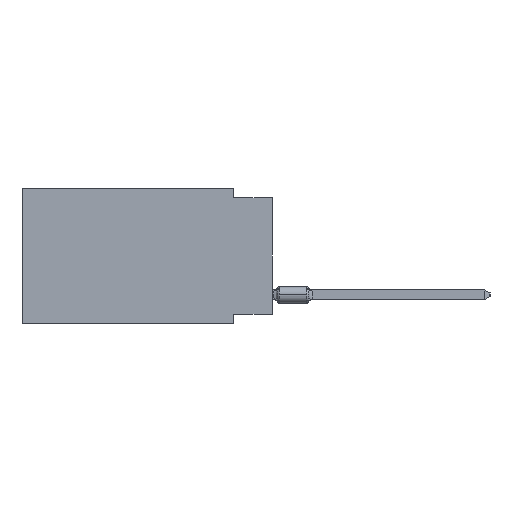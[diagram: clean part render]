
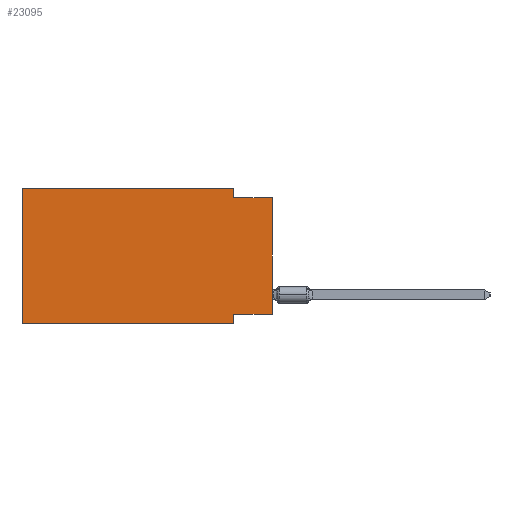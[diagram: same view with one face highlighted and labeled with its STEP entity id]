
A CAD part, left-side view. The second image highlights one B-rep face of the part: STEP entity #23095.
In plain terms, the highlighted planar face has unit normal (-1, 0, 0).
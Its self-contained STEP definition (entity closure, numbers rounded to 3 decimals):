
#144 = EDGE_CURVE ( 'NONE', #15184, #32745, #8594, .T. ) ;
#455 = ORIENTED_EDGE ( 'NONE', *, *, #16680, .F. ) ;
#2168 = ORIENTED_EDGE ( 'NONE', *, *, #20220, .F. ) ;
#2653 = CARTESIAN_POINT ( 'NONE',  ( 0., 0., -0.635 ) ) ;
#5180 = LINE ( 'NONE', #40869, #28693 ) ;
#6357 = ORIENTED_EDGE ( 'NONE', *, *, #12459, .T. ) ;
#7668 = DIRECTION ( 'NONE',  ( 0., 0., -1. ) ) ;
#8041 = ORIENTED_EDGE ( 'NONE', *, *, #144, .F. ) ;
#8301 = CARTESIAN_POINT ( 'NONE',  ( 0., 16.383, 0. ) ) ;
#8594 = LINE ( 'NONE', #16856, #38137 ) ;
#9159 = LINE ( 'NONE', #21857, #26426 ) ;
#9994 = VERTEX_POINT ( 'NONE', #51847 ) ;
#10965 = VECTOR ( 'NONE', #41348, 1000. ) ;
#11211 = CARTESIAN_POINT ( 'NONE',  ( 0., 2.54, 0. ) ) ;
#11856 = VERTEX_POINT ( 'NONE', #39133 ) ;
#12459 = EDGE_CURVE ( 'NONE', #15184, #53802, #41325, .T. ) ;
#12996 = DIRECTION ( 'NONE',  ( 0., 0., -1. ) ) ;
#15184 = VERTEX_POINT ( 'NONE', #36613 ) ;
#15350 = EDGE_LOOP ( 'NONE', ( #41732, #2168, #28341, #30673, #8041, #6357, #15397, #455 ) ) ;
#15397 = ORIENTED_EDGE ( 'NONE', *, *, #29997, .F. ) ;
#15806 = CARTESIAN_POINT ( 'NONE',  ( 0., 0., -8.255 ) ) ;
#16680 = EDGE_CURVE ( 'NONE', #45588, #11856, #53089, .T. ) ;
#16856 = CARTESIAN_POINT ( 'NONE',  ( 0., 16.383, 0. ) ) ;
#17795 = VECTOR ( 'NONE', #7668, 1000. ) ;
#18474 = AXIS2_PLACEMENT_3D ( 'NONE', #33697, #32548, #50539 ) ;
#18913 = DIRECTION ( 'NONE',  ( 0., -1., 0. ) ) ;
#20220 = EDGE_CURVE ( 'NONE', #9994, #50103, #5180, .T. ) ;
#21504 = VECTOR ( 'NONE', #18913, 1000. ) ;
#21857 = CARTESIAN_POINT ( 'NONE',  ( 0., 2.54, -8.89 ) ) ;
#21991 = CARTESIAN_POINT ( 'NONE',  ( 0., 2.54, 0. ) ) ;
#22128 = DIRECTION ( 'NONE',  ( 0., 1., 0. ) ) ;
#23095 = ADVANCED_FACE ( 'NONE', ( #55823 ), #23418, .F. ) ;
#23418 = PLANE ( 'NONE',  #18474 ) ;
#23949 = LINE ( 'NONE', #45471, #10965 ) ;
#26426 = VECTOR ( 'NONE', #12996, 1000. ) ;
#26551 = CARTESIAN_POINT ( 'NONE',  ( 0., 0., -8.255 ) ) ;
#27230 = EDGE_CURVE ( 'NONE', #45695, #9994, #56624, .T. ) ;
#27297 = CARTESIAN_POINT ( 'NONE',  ( 0., 0., 0. ) ) ;
#28169 = DIRECTION ( 'NONE',  ( 0., -1., 0. ) ) ;
#28341 = ORIENTED_EDGE ( 'NONE', *, *, #27230, .F. ) ;
#28693 = VECTOR ( 'NONE', #28169, 1000. ) ;
#29997 = EDGE_CURVE ( 'NONE', #11856, #53802, #9159, .T. ) ;
#30673 = ORIENTED_EDGE ( 'NONE', *, *, #43384, .F. ) ;
#30845 = DIRECTION ( 'NONE',  ( 0., 0., 1. ) ) ;
#31423 = LINE ( 'NONE', #27297, #57673 ) ;
#32055 = VECTOR ( 'NONE', #22128, 1000. ) ;
#32548 = DIRECTION ( 'NONE',  ( 1., 0., 0. ) ) ;
#32745 = VERTEX_POINT ( 'NONE', #8301 ) ;
#33697 = CARTESIAN_POINT ( 'NONE',  ( 0., 16.383, 0. ) ) ;
#36613 = CARTESIAN_POINT ( 'NONE',  ( 0., 16.383, -8.89 ) ) ;
#38137 = VECTOR ( 'NONE', #53715, 1000. ) ;
#39133 = CARTESIAN_POINT ( 'NONE',  ( 0., 2.54, -8.255 ) ) ;
#40869 = CARTESIAN_POINT ( 'NONE',  ( 0., 0., -0.635 ) ) ;
#41325 = LINE ( 'NONE', #51324, #21504 ) ;
#41348 = DIRECTION ( 'NONE',  ( 0., -1., 0. ) ) ;
#41732 = ORIENTED_EDGE ( 'NONE', *, *, #46974, .T. ) ;
#43384 = EDGE_CURVE ( 'NONE', #32745, #45695, #23949, .T. ) ;
#45471 = CARTESIAN_POINT ( 'NONE',  ( 0., 16.383, 0. ) ) ;
#45588 = VERTEX_POINT ( 'NONE', #15806 ) ;
#45695 = VERTEX_POINT ( 'NONE', #21991 ) ;
#46974 = EDGE_CURVE ( 'NONE', #45588, #50103, #31423, .T. ) ;
#50103 = VERTEX_POINT ( 'NONE', #2653 ) ;
#50539 = DIRECTION ( 'NONE',  ( 0., 0., -1. ) ) ;
#51324 = CARTESIAN_POINT ( 'NONE',  ( 0., 16.383, -8.89 ) ) ;
#51847 = CARTESIAN_POINT ( 'NONE',  ( 0., 2.54, -0.635 ) ) ;
#53089 = LINE ( 'NONE', #26551, #32055 ) ;
#53715 = DIRECTION ( 'NONE',  ( 0., 0., 1. ) ) ;
#53802 = VERTEX_POINT ( 'NONE', #55921 ) ;
#55823 = FACE_OUTER_BOUND ( 'NONE', #15350, .T. ) ;
#55921 = CARTESIAN_POINT ( 'NONE',  ( 0., 2.54, -8.89 ) ) ;
#56624 = LINE ( 'NONE', #11211, #17795 ) ;
#57673 = VECTOR ( 'NONE', #30845, 1000. ) ;
